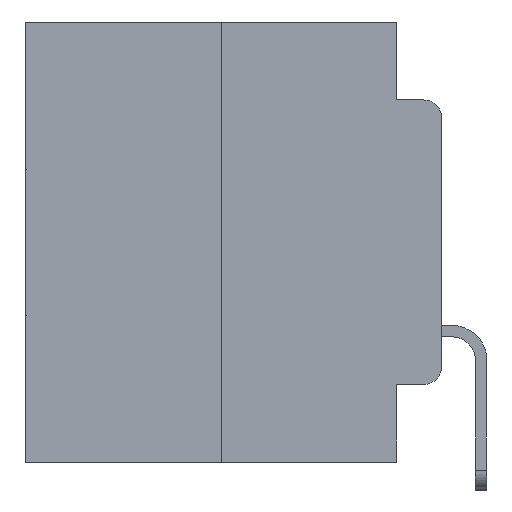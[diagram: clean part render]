
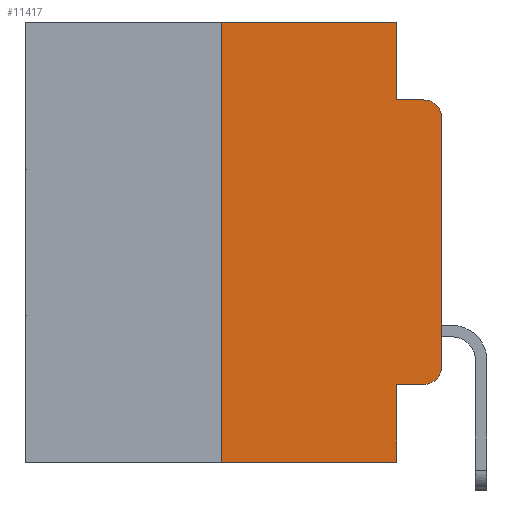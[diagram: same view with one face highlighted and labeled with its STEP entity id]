
A CAD part, left-side view. The second image highlights one B-rep face of the part: STEP entity #11417.
In plain terms, the highlighted planar face has unit normal (-1, 0, 0).
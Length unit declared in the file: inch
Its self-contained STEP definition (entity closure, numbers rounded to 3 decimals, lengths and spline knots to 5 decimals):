
#167 = EDGE_CURVE ( 'NONE', #3721, #27508, #17352, .T. ) ;
#853 = DIRECTION ( 'NONE',  ( 0., -1., 0. ) ) ;
#1105 = DIRECTION ( 'NONE',  ( 0., 0., -1. ) ) ;
#1317 = VECTOR ( 'NONE', #26611, 39.37008 ) ;
#1449 = PLANE ( 'NONE',  #4521 ) ;
#1646 = CIRCLE ( 'NONE', #19588, 0.02 ) ;
#2425 = LINE ( 'NONE', #25036, #11385 ) ;
#2462 = DIRECTION ( 'NONE',  ( 0., 0., -1. ) ) ;
#3127 = CARTESIAN_POINT ( 'NONE',  ( 0., 0.25, 0. ) ) ;
#3539 = VECTOR ( 'NONE', #853, 39.37008 ) ;
#3590 = EDGE_CURVE ( 'NONE', #9935, #8092, #14398, .T. ) ;
#3721 = VERTEX_POINT ( 'NONE', #5244 ) ;
#3861 = DIRECTION ( 'NONE',  ( 1., 0., 0. ) ) ;
#3952 = VECTOR ( 'NONE', #9594, 39.37008 ) ;
#4098 = LINE ( 'NONE', #15459, #1317 ) ;
#4521 = AXIS2_PLACEMENT_3D ( 'NONE', #18966, #3861, #25870 ) ;
#4553 = VERTEX_POINT ( 'NONE', #17028 ) ;
#4978 = CARTESIAN_POINT ( 'NONE',  ( 0., 0.25, 0. ) ) ;
#5244 = CARTESIAN_POINT ( 'NONE',  ( 0., 0., -0.3915 ) ) ;
#5269 = LINE ( 'NONE', #27211, #25211 ) ;
#5662 = DIRECTION ( 'NONE',  ( -1., 0., 0. ) ) ;
#6098 = CARTESIAN_POINT ( 'NONE',  ( 0., 0., 0. ) ) ;
#7551 = EDGE_CURVE ( 'NONE', #9935, #15866, #26600, .T. ) ;
#7917 = ORIENTED_EDGE ( 'NONE', *, *, #27712, .F. ) ;
#8092 = VERTEX_POINT ( 'NONE', #15846 ) ;
#8548 = VECTOR ( 'NONE', #2462, 39.37008 ) ;
#8644 = VECTOR ( 'NONE', #21687, 39.37008 ) ;
#8708 = EDGE_CURVE ( 'NONE', #27508, #4553, #19284, .T. ) ;
#9528 = CARTESIAN_POINT ( 'NONE',  ( 0., 0.02, -0.4115 ) ) ;
#9594 = DIRECTION ( 'NONE',  ( 0., 0., 1. ) ) ;
#9626 = AXIS2_PLACEMENT_3D ( 'NONE', #16377, #27141, #18123 ) ;
#9935 = VERTEX_POINT ( 'NONE', #22184 ) ;
#10418 = DIRECTION ( 'NONE',  ( 0., 0., 1. ) ) ;
#10835 = VERTEX_POINT ( 'NONE', #23173 ) ;
#11024 = ORIENTED_EDGE ( 'NONE', *, *, #19753, .T. ) ;
#11114 = VERTEX_POINT ( 'NONE', #15982 ) ;
#11385 = VECTOR ( 'NONE', #1105, 39.37008 ) ;
#11417 = ADVANCED_FACE ( 'NONE', ( #13280 ), #1449, .F. ) ;
#11540 = ORIENTED_EDGE ( 'NONE', *, *, #167, .T. ) ;
#11604 = CARTESIAN_POINT ( 'NONE',  ( 0., 0.051, 0. ) ) ;
#11710 = CARTESIAN_POINT ( 'NONE',  ( 0., 0., -0.1085 ) ) ;
#12223 = ORIENTED_EDGE ( 'NONE', *, *, #8708, .T. ) ;
#13280 = FACE_OUTER_BOUND ( 'NONE', #22057, .T. ) ;
#13963 = ORIENTED_EDGE ( 'NONE', *, *, #7551, .T. ) ;
#14065 = CARTESIAN_POINT ( 'NONE',  ( 0., 0.051, -0.4115 ) ) ;
#14165 = EDGE_CURVE ( 'NONE', #18132, #10835, #4098, .T. ) ;
#14398 = LINE ( 'NONE', #11604, #8548 ) ;
#15191 = LINE ( 'NONE', #26134, #8644 ) ;
#15317 = ORIENTED_EDGE ( 'NONE', *, *, #14165, .F. ) ;
#15459 = CARTESIAN_POINT ( 'NONE',  ( 0., 0.473, 0. ) ) ;
#15633 = LINE ( 'NONE', #3127, #3952 ) ;
#15846 = CARTESIAN_POINT ( 'NONE',  ( 0., 0.051, -0.5 ) ) ;
#15866 = VERTEX_POINT ( 'NONE', #9528 ) ;
#15982 = CARTESIAN_POINT ( 'NONE',  ( 0., 0.25, -0.5 ) ) ;
#16377 = CARTESIAN_POINT ( 'NONE',  ( 0., 0.02, -0.1085 ) ) ;
#16659 = VECTOR ( 'NONE', #10418, 39.37008 ) ;
#17028 = CARTESIAN_POINT ( 'NONE',  ( 0., 0.02, -0.0885 ) ) ;
#17352 = LINE ( 'NONE', #6098, #16659 ) ;
#17720 = ORIENTED_EDGE ( 'NONE', *, *, #21841, .F. ) ;
#18123 = DIRECTION ( 'NONE',  ( 0., 0., -1. ) ) ;
#18132 = VERTEX_POINT ( 'NONE', #4978 ) ;
#18966 = CARTESIAN_POINT ( 'NONE',  ( 0., 0.473, 0. ) ) ;
#19284 = CIRCLE ( 'NONE', #9626, 0.02 ) ;
#19588 = AXIS2_PLACEMENT_3D ( 'NONE', #27474, #5662, #21016 ) ;
#19753 = EDGE_CURVE ( 'NONE', #15866, #3721, #1646, .T. ) ;
#19767 = ORIENTED_EDGE ( 'NONE', *, *, #3590, .F. ) ;
#21016 = DIRECTION ( 'NONE',  ( 0., 0., -1. ) ) ;
#21687 = DIRECTION ( 'NONE',  ( 0., -1., 0. ) ) ;
#21841 = EDGE_CURVE ( 'NONE', #11114, #18132, #15633, .T. ) ;
#22057 = EDGE_LOOP ( 'NONE', ( #11540, #12223, #27767, #7917, #15317, #17720, #25151, #19767, #13963, #11024 ) ) ;
#22184 = CARTESIAN_POINT ( 'NONE',  ( 0., 0.051, -0.4115 ) ) ;
#22538 = EDGE_CURVE ( 'NONE', #11114, #8092, #5269, .T. ) ;
#22764 = DIRECTION ( 'NONE',  ( 0., -1., 0. ) ) ;
#23173 = CARTESIAN_POINT ( 'NONE',  ( 0., 0.051, 0. ) ) ;
#23937 = EDGE_CURVE ( 'NONE', #24339, #4553, #15191, .T. ) ;
#24339 = VERTEX_POINT ( 'NONE', #27542 ) ;
#25036 = CARTESIAN_POINT ( 'NONE',  ( 0., 0.051, 0. ) ) ;
#25151 = ORIENTED_EDGE ( 'NONE', *, *, #22538, .T. ) ;
#25211 = VECTOR ( 'NONE', #22764, 39.37008 ) ;
#25870 = DIRECTION ( 'NONE',  ( 0., 0., -1. ) ) ;
#26134 = CARTESIAN_POINT ( 'NONE',  ( 0., 0.051, -0.0885 ) ) ;
#26600 = LINE ( 'NONE', #14065, #3539 ) ;
#26611 = DIRECTION ( 'NONE',  ( 0., -1., 0. ) ) ;
#27141 = DIRECTION ( 'NONE',  ( -1., 0., 0. ) ) ;
#27211 = CARTESIAN_POINT ( 'NONE',  ( 0., 0.473, -0.5 ) ) ;
#27474 = CARTESIAN_POINT ( 'NONE',  ( 0., 0.02, -0.3915 ) ) ;
#27508 = VERTEX_POINT ( 'NONE', #11710 ) ;
#27542 = CARTESIAN_POINT ( 'NONE',  ( 0., 0.051, -0.0885 ) ) ;
#27712 = EDGE_CURVE ( 'NONE', #10835, #24339, #2425, .T. ) ;
#27767 = ORIENTED_EDGE ( 'NONE', *, *, #23937, .F. ) ;
